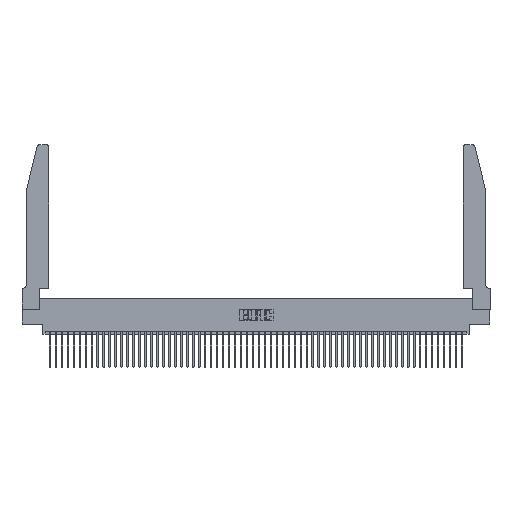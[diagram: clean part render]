
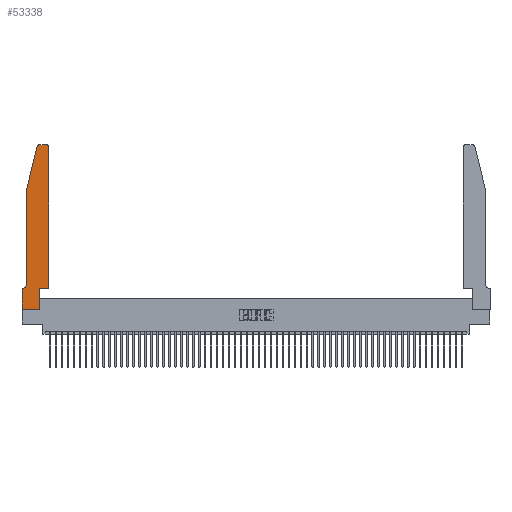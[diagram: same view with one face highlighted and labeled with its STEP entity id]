
A CAD part, top view. The second image highlights one B-rep face of the part: STEP entity #53338.
In plain terms, the highlighted planar face has unit normal (0, 0, 1).
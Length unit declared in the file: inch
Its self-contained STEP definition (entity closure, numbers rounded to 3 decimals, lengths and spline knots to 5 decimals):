
#1398 = EDGE_CURVE ( 'NONE', #46263, #38541, #28005, .T. ) ;
#1407 = EDGE_CURVE ( 'NONE', #20396, #5747, #4920, .T. ) ;
#1667 = AXIS2_PLACEMENT_3D ( 'NONE', #28162, #2126, #32515 ) ;
#2126 = DIRECTION ( 'NONE',  ( 0., 0., 1. ) ) ;
#2947 = DIRECTION ( 'NONE',  ( -1., 0., 0. ) ) ;
#3931 = DIRECTION ( 'NONE',  ( -1., 0., 0. ) ) ;
#4617 = VERTEX_POINT ( 'NONE', #12803 ) ;
#4920 = LINE ( 'NONE', #25108, #38171 ) ;
#5341 = LINE ( 'NONE', #15943, #50046 ) ;
#5747 = VERTEX_POINT ( 'NONE', #28390 ) ;
#5961 = LINE ( 'NONE', #46552, #30405 ) ;
#6570 = VECTOR ( 'NONE', #42935, 39.37008 ) ;
#6634 = CARTESIAN_POINT ( 'NONE',  ( 0.4505, 0.35, 0.37 ) ) ;
#6796 = ORIENTED_EDGE ( 'NONE', *, *, #1407, .T. ) ;
#7019 = VECTOR ( 'NONE', #40204, 39.37008 ) ;
#7346 = ORIENTED_EDGE ( 'NONE', *, *, #46296, .T. ) ;
#9105 = CARTESIAN_POINT ( 'NONE',  ( 0.0755, 2., 0.37 ) ) ;
#9200 = CARTESIAN_POINT ( 'NONE',  ( 0., 0.35, 0.37 ) ) ;
#10204 = CARTESIAN_POINT ( 'NONE',  ( 0.2865, 0.35, 0.37 ) ) ;
#10567 = CARTESIAN_POINT ( 'NONE',  ( 0.4205, 2.75, 0.37 ) ) ;
#10760 = FACE_OUTER_BOUND ( 'NONE', #45521, .T. ) ;
#10800 = CARTESIAN_POINT ( 'NONE',  ( 0.4205, 2.72, 0.37 ) ) ;
#11018 = DIRECTION ( 'NONE',  ( 1., 0., 0. ) ) ;
#11063 = VECTOR ( 'NONE', #11018, 39.37008 ) ;
#11244 = ORIENTED_EDGE ( 'NONE', *, *, #21166, .T. ) ;
#11841 = VERTEX_POINT ( 'NONE', #36573 ) ;
#12068 = CARTESIAN_POINT ( 'NONE',  ( 0.4505, 0.35, 0.37 ) ) ;
#12345 = VERTEX_POINT ( 'NONE', #10204 ) ;
#12523 = ORIENTED_EDGE ( 'NONE', *, *, #38660, .T. ) ;
#12678 = VECTOR ( 'NONE', #14084, 39.37008 ) ;
#12803 = CARTESIAN_POINT ( 'NONE',  ( 0.25487, 2.72718, 0.37 ) ) ;
#12821 = EDGE_CURVE ( 'NONE', #11841, #55994, #5341, .T. ) ;
#13572 = PLANE ( 'NONE',  #32231 ) ;
#14084 = DIRECTION ( 'NONE',  ( 0., 1., 0. ) ) ;
#15194 = DIRECTION ( 'NONE',  ( 1., 0., 0. ) ) ;
#15255 = EDGE_CURVE ( 'NONE', #40460, #4617, #54468, .T. ) ;
#15943 = CARTESIAN_POINT ( 'NONE',  ( 0.0755, 0.35, 0.37 ) ) ;
#16503 = EDGE_CURVE ( 'NONE', #5747, #11841, #33945, .T. ) ;
#18139 = LINE ( 'NONE', #25555, #6570 ) ;
#20396 = VERTEX_POINT ( 'NONE', #9105 ) ;
#21166 = EDGE_CURVE ( 'NONE', #33486, #44125, #41559, .T. ) ;
#22276 = DIRECTION ( 'NONE',  ( 1., 0., 0. ) ) ;
#22591 = LINE ( 'NONE', #6634, #11063 ) ;
#24662 = AXIS2_PLACEMENT_3D ( 'NONE', #55763, #29931, #3931 ) ;
#24704 = CARTESIAN_POINT ( 'NONE',  ( 0., 0., 0.37 ) ) ;
#25108 = CARTESIAN_POINT ( 'NONE',  ( 0.0755, 2., 0.37 ) ) ;
#25303 = CARTESIAN_POINT ( 'NONE',  ( 0., 0.35, 0.37 ) ) ;
#25363 = VECTOR ( 'NONE', #33423, 39.37008 ) ;
#25555 = CARTESIAN_POINT ( 'NONE',  ( 0., 0., 0.37 ) ) ;
#25911 = ORIENTED_EDGE ( 'NONE', *, *, #1398, .T. ) ;
#26904 = CARTESIAN_POINT ( 'NONE',  ( 0.2865, 0.35, 0.37 ) ) ;
#28005 = LINE ( 'NONE', #12068, #39483 ) ;
#28103 = ORIENTED_EDGE ( 'NONE', *, *, #33919, .T. ) ;
#28162 = CARTESIAN_POINT ( 'NONE',  ( 0.284, 2.72, 0.37 ) ) ;
#28390 = CARTESIAN_POINT ( 'NONE',  ( 0.0755, 0.42, 0.37 ) ) ;
#28985 = CARTESIAN_POINT ( 'NONE',  ( 0.4505, 2.72, 0.37 ) ) ;
#29269 = CIRCLE ( 'NONE', #48329, 0.03 ) ;
#29401 = DIRECTION ( 'NONE',  ( -0.239, -0.971, 0. ) ) ;
#29931 = DIRECTION ( 'NONE',  ( 0., 0., -1. ) ) ;
#30405 = VECTOR ( 'NONE', #29401, 39.37008 ) ;
#30468 = CARTESIAN_POINT ( 'NONE',  ( 0.284, 2.75, 0.37 ) ) ;
#30737 = VERTEX_POINT ( 'NONE', #10567 ) ;
#32231 = AXIS2_PLACEMENT_3D ( 'NONE', #9200, #48109, #22276 ) ;
#32291 = ORIENTED_EDGE ( 'NONE', *, *, #12821, .T. ) ;
#32515 = DIRECTION ( 'NONE',  ( 1., 0., 0. ) ) ;
#32910 = ORIENTED_EDGE ( 'NONE', *, *, #15255, .T. ) ;
#33423 = DIRECTION ( 'NONE',  ( -1., 0., 0. ) ) ;
#33486 = VERTEX_POINT ( 'NONE', #24704 ) ;
#33629 = DIRECTION ( 'NONE',  ( 0., 1., 0. ) ) ;
#33919 = EDGE_CURVE ( 'NONE', #4617, #20396, #5961, .T. ) ;
#33945 = CIRCLE ( 'NONE', #24662, 0.07 ) ;
#35697 = LINE ( 'NONE', #26904, #12678 ) ;
#35736 = ORIENTED_EDGE ( 'NONE', *, *, #45819, .T. ) ;
#35924 = CARTESIAN_POINT ( 'NONE',  ( 0., 0., 0.37 ) ) ;
#36220 = EDGE_CURVE ( 'NONE', #38541, #30737, #29269, .T. ) ;
#36573 = CARTESIAN_POINT ( 'NONE',  ( 0.0055, 0.35, 0.37 ) ) ;
#37079 = ORIENTED_EDGE ( 'NONE', *, *, #36220, .T. ) ;
#38171 = VECTOR ( 'NONE', #55312, 39.37008 ) ;
#38541 = VERTEX_POINT ( 'NONE', #28985 ) ;
#38660 = EDGE_CURVE ( 'NONE', #55994, #33486, #18139, .T. ) ;
#39483 = VECTOR ( 'NONE', #33629, 39.37008 ) ;
#39893 = EDGE_CURVE ( 'NONE', #44125, #12345, #35697, .T. ) ;
#40204 = DIRECTION ( 'NONE',  ( 1., 0., 0. ) ) ;
#40460 = VERTEX_POINT ( 'NONE', #30468 ) ;
#40953 = ORIENTED_EDGE ( 'NONE', *, *, #16503, .T. ) ;
#41054 = DIRECTION ( 'NONE',  ( 0., 0., 1. ) ) ;
#41559 = LINE ( 'NONE', #35924, #7019 ) ;
#42935 = DIRECTION ( 'NONE',  ( 0., -1., 0. ) ) ;
#44125 = VERTEX_POINT ( 'NONE', #47114 ) ;
#45521 = EDGE_LOOP ( 'NONE', ( #35736, #32910, #28103, #6796, #40953, #32291, #12523, #11244, #55236, #7346, #25911, #37079 ) ) ;
#45819 = EDGE_CURVE ( 'NONE', #30737, #40460, #46959, .T. ) ;
#46263 = VERTEX_POINT ( 'NONE', #53740 ) ;
#46296 = EDGE_CURVE ( 'NONE', #12345, #46263, #22591, .T. ) ;
#46396 = CARTESIAN_POINT ( 'NONE',  ( 0.2605, 2.75, 0.37 ) ) ;
#46552 = CARTESIAN_POINT ( 'NONE',  ( 0.0755, 2., 0.37 ) ) ;
#46959 = LINE ( 'NONE', #46396, #25363 ) ;
#47114 = CARTESIAN_POINT ( 'NONE',  ( 0.2865, 0., 0.37 ) ) ;
#48109 = DIRECTION ( 'NONE',  ( 0., 0., 1. ) ) ;
#48329 = AXIS2_PLACEMENT_3D ( 'NONE', #10800, #41054, #15194 ) ;
#50046 = VECTOR ( 'NONE', #2947, 39.37008 ) ;
#53338 = ADVANCED_FACE ( 'NONE', ( #10760 ), #13572, .T. ) ;
#53740 = CARTESIAN_POINT ( 'NONE',  ( 0.4505, 0.35, 0.37 ) ) ;
#54468 = CIRCLE ( 'NONE', #1667, 0.03 ) ;
#55236 = ORIENTED_EDGE ( 'NONE', *, *, #39893, .T. ) ;
#55312 = DIRECTION ( 'NONE',  ( 0., -1., 0. ) ) ;
#55763 = CARTESIAN_POINT ( 'NONE',  ( 0.0055, 0.42, 0.37 ) ) ;
#55994 = VERTEX_POINT ( 'NONE', #25303 ) ;
